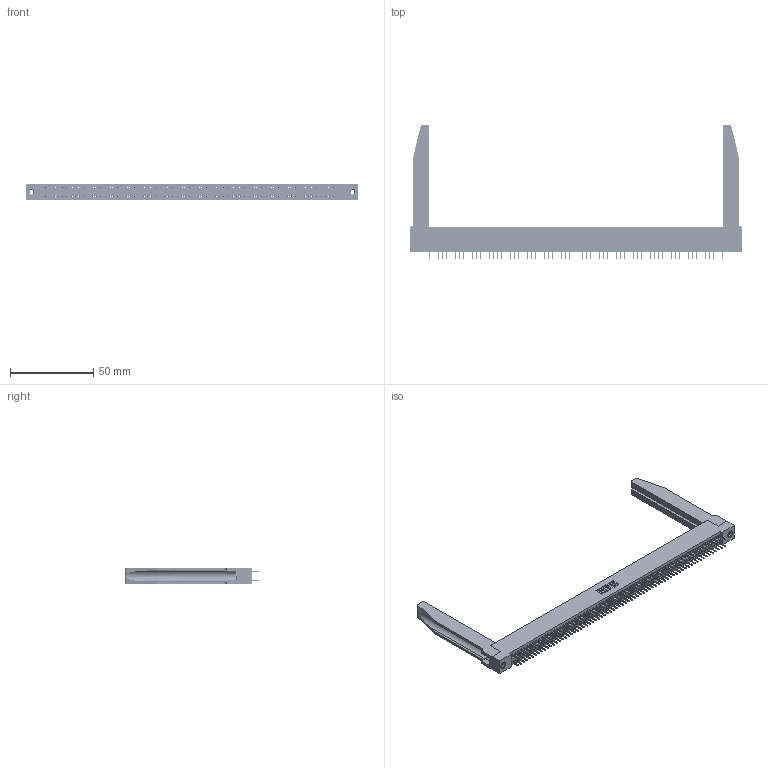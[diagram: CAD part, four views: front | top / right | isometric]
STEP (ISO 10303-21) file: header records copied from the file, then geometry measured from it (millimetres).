
FILE_DESCRIPTION (( 'STEP AP203' ), '1' );
FILE_NAME ('345-140-524-278.STEP', '2019-11-08T20:22:48', ( '' ), ( '' ), 'SwSTEP 2.0', 'SolidWorks 2016', '' );
FILE_SCHEMA (( 'CONFIG_CONTROL_DESIGN' ));
Length unit declared in the file: inch
Products named in the file (5): 345 Part_Flush Mounting Lugs - 0.156 Dia-TH; 345-292-001_345-293-124; 345-220-078_345-220-078; 345-250-001_345-250-001-102; 345-140-524-278
Assembly tree (145 placements, depth 2):
  345-140-524-278
    345 Part_Flush Mounting Lugs - 0.156 Dia-TH
    345-292-001_345-293-124  x140
    345-250-001_345-250-001-102  x2
    345-220-078_345-220-078  x2
Bounding box: 199.03 x 80.31 x 9.4 mm (x, y, z)
Volume: 27152.9 mm3; surface area: 35472 mm2
Topology: 145 solids, 145 shells, 7920 faces, 22369 edges, 14342 vertices
Faces by surface type: plane 5682, cylinder 2186, bspline 36, cone 12, torus 4
Entity records: 55968 total; most frequent: CARTESIAN_POINT 10271, ORIENTED_EDGE 9102, DIRECTION 8017, EDGE_CURVE 4551, VECTOR 4049, LINE 4049, VERTEX_POINT 3024, AXIS2_PLACEMENT_3D 1984
